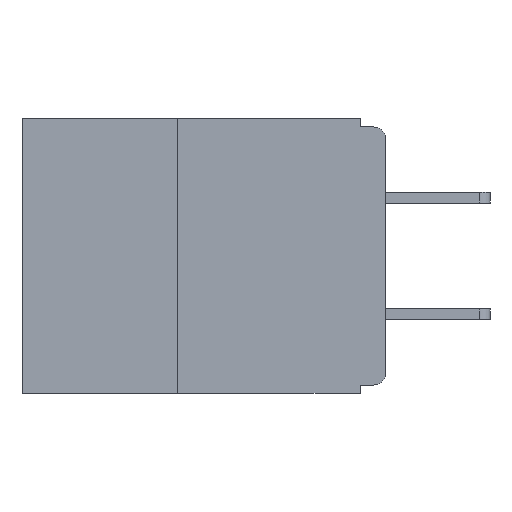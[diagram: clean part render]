
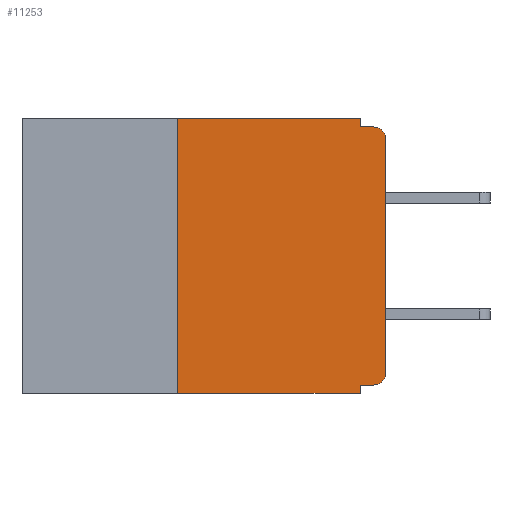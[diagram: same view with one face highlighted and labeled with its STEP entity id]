
A CAD part, left-side view. The second image highlights one B-rep face of the part: STEP entity #11253.
In plain terms, the highlighted planar face has unit normal (-1, 0, 0).
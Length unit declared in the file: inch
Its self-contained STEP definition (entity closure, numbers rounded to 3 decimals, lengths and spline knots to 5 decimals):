
#102 = PLANE ( 'NONE',  #2781 ) ;
#199 = LINE ( 'NONE', #8749, #9888 ) ;
#378 = VERTEX_POINT ( 'NONE', #8535 ) ;
#461 = DIRECTION ( 'NONE',  ( -1., 0., 0. ) ) ;
#949 = EDGE_CURVE ( 'NONE', #5296, #9739, #12465, .T. ) ;
#1408 = CARTESIAN_POINT ( 'NONE',  ( 0., 0.25, -0.33 ) ) ;
#2307 = VERTEX_POINT ( 'NONE', #14805 ) ;
#2368 = EDGE_CURVE ( 'NONE', #4282, #378, #5229, .T. ) ;
#2715 = DIRECTION ( 'NONE',  ( 1., 0., 0. ) ) ;
#2781 = AXIS2_PLACEMENT_3D ( 'NONE', #10385, #2715, #11655 ) ;
#2796 = DIRECTION ( 'NONE',  ( 0., 0., -1. ) ) ;
#2824 = ORIENTED_EDGE ( 'NONE', *, *, #14196, .T. ) ;
#3246 = DIRECTION ( 'NONE',  ( 0., 1., 0. ) ) ;
#3349 = LINE ( 'NONE', #10848, #5934 ) ;
#3844 = VERTEX_POINT ( 'NONE', #15344 ) ;
#4154 = ORIENTED_EDGE ( 'NONE', *, *, #13032, .F. ) ;
#4282 = VERTEX_POINT ( 'NONE', #16244 ) ;
#4456 = DIRECTION ( 'NONE',  ( 0., -1., 0. ) ) ;
#4633 = VERTEX_POINT ( 'NONE', #6848 ) ;
#4854 = DIRECTION ( 'NONE',  ( 0., 0., -1. ) ) ;
#5229 = LINE ( 'NONE', #14858, #14557 ) ;
#5243 = CARTESIAN_POINT ( 'NONE',  ( 0., 0.015, -0.01 ) ) ;
#5296 = VERTEX_POINT ( 'NONE', #5689 ) ;
#5303 = EDGE_CURVE ( 'NONE', #12969, #7593, #3349, .T. ) ;
#5328 = EDGE_CURVE ( 'NONE', #3844, #7593, #15642, .T. ) ;
#5333 = AXIS2_PLACEMENT_3D ( 'NONE', #13406, #5808, #14674 ) ;
#5508 = CARTESIAN_POINT ( 'NONE',  ( 0., 0., 0. ) ) ;
#5681 = VECTOR ( 'NONE', #3246, 39.37008 ) ;
#5689 = CARTESIAN_POINT ( 'NONE',  ( 0., 0.015, -0.32 ) ) ;
#5754 = EDGE_CURVE ( 'NONE', #2307, #3844, #10157, .T. ) ;
#5756 = EDGE_CURVE ( 'NONE', #5296, #2307, #9754, .T. ) ;
#5808 = DIRECTION ( 'NONE',  ( -1., 0., 0. ) ) ;
#5930 = LINE ( 'NONE', #1408, #14852 ) ;
#5934 = VECTOR ( 'NONE', #4456, 39.37008 ) ;
#6339 = ORIENTED_EDGE ( 'NONE', *, *, #5328, .T. ) ;
#6848 = CARTESIAN_POINT ( 'NONE',  ( 0., 0.25, -0.33 ) ) ;
#7117 = VERTEX_POINT ( 'NONE', #14474 ) ;
#7417 = EDGE_CURVE ( 'NONE', #9739, #7117, #199, .T. ) ;
#7593 = VERTEX_POINT ( 'NONE', #5243 ) ;
#7788 = DIRECTION ( 'NONE',  ( 0., 0., 1. ) ) ;
#8160 = CARTESIAN_POINT ( 'NONE',  ( 0., 0.015, -0.305 ) ) ;
#8238 = ORIENTED_EDGE ( 'NONE', *, *, #5754, .T. ) ;
#8301 = LINE ( 'NONE', #15216, #11297 ) ;
#8535 = CARTESIAN_POINT ( 'NONE',  ( 0., 0.031, 0. ) ) ;
#8749 = CARTESIAN_POINT ( 'NONE',  ( 0., 0.031, -0.33 ) ) ;
#8922 = VECTOR ( 'NONE', #2796, 39.37008 ) ;
#8944 = DIRECTION ( 'NONE',  ( 0., -1., 0. ) ) ;
#9463 = DIRECTION ( 'NONE',  ( 0., 0., -1. ) ) ;
#9546 = ORIENTED_EDGE ( 'NONE', *, *, #2368, .F. ) ;
#9640 = ORIENTED_EDGE ( 'NONE', *, *, #949, .F. ) ;
#9739 = VERTEX_POINT ( 'NONE', #13475 ) ;
#9754 = CIRCLE ( 'NONE', #13547, 0.015 ) ;
#9888 = VECTOR ( 'NONE', #4854, 39.37008 ) ;
#10157 = LINE ( 'NONE', #5508, #12693 ) ;
#10385 = CARTESIAN_POINT ( 'NONE',  ( 0., 0.437, 0. ) ) ;
#10848 = CARTESIAN_POINT ( 'NONE',  ( 0., 0., -0.01 ) ) ;
#11253 = ADVANCED_FACE ( 'NONE', ( #12499 ), #102, .F. ) ;
#11297 = VECTOR ( 'NONE', #8944, 39.37008 ) ;
#11655 = DIRECTION ( 'NONE',  ( 0., 0., -1. ) ) ;
#11899 = EDGE_CURVE ( 'NONE', #378, #12969, #12277, .T. ) ;
#12164 = CARTESIAN_POINT ( 'NONE',  ( 0., 0., -0.32 ) ) ;
#12277 = LINE ( 'NONE', #14184, #8922 ) ;
#12344 = DIRECTION ( 'NONE',  ( 0., -1., 0. ) ) ;
#12465 = LINE ( 'NONE', #12164, #5681 ) ;
#12499 = FACE_OUTER_BOUND ( 'NONE', #13841, .T. ) ;
#12693 = VECTOR ( 'NONE', #13183, 39.37008 ) ;
#12730 = CARTESIAN_POINT ( 'NONE',  ( 0., 0.031, -0.01 ) ) ;
#12969 = VERTEX_POINT ( 'NONE', #12730 ) ;
#13032 = EDGE_CURVE ( 'NONE', #4633, #4282, #5930, .T. ) ;
#13183 = DIRECTION ( 'NONE',  ( 0., 0., 1. ) ) ;
#13406 = CARTESIAN_POINT ( 'NONE',  ( 0., 0.015, -0.025 ) ) ;
#13475 = CARTESIAN_POINT ( 'NONE',  ( 0., 0.031, -0.32 ) ) ;
#13547 = AXIS2_PLACEMENT_3D ( 'NONE', #8160, #461, #9463 ) ;
#13810 = ORIENTED_EDGE ( 'NONE', *, *, #11899, .F. ) ;
#13841 = EDGE_LOOP ( 'NONE', ( #8238, #6339, #15470, #13810, #9546, #4154, #2824, #14472, #9640, #15766 ) ) ;
#14184 = CARTESIAN_POINT ( 'NONE',  ( 0., 0.031, 0. ) ) ;
#14196 = EDGE_CURVE ( 'NONE', #4633, #7117, #8301, .T. ) ;
#14472 = ORIENTED_EDGE ( 'NONE', *, *, #7417, .F. ) ;
#14474 = CARTESIAN_POINT ( 'NONE',  ( 0., 0.031, -0.33 ) ) ;
#14557 = VECTOR ( 'NONE', #12344, 39.37008 ) ;
#14674 = DIRECTION ( 'NONE',  ( 0., 0., -1. ) ) ;
#14805 = CARTESIAN_POINT ( 'NONE',  ( 0., 0., -0.305 ) ) ;
#14852 = VECTOR ( 'NONE', #7788, 39.37008 ) ;
#14858 = CARTESIAN_POINT ( 'NONE',  ( 0., 0.437, 0. ) ) ;
#15216 = CARTESIAN_POINT ( 'NONE',  ( 0., 0.437, -0.33 ) ) ;
#15344 = CARTESIAN_POINT ( 'NONE',  ( 0., 0., -0.025 ) ) ;
#15470 = ORIENTED_EDGE ( 'NONE', *, *, #5303, .F. ) ;
#15642 = CIRCLE ( 'NONE', #5333, 0.015 ) ;
#15766 = ORIENTED_EDGE ( 'NONE', *, *, #5756, .T. ) ;
#16244 = CARTESIAN_POINT ( 'NONE',  ( 0., 0.25, 0. ) ) ;
